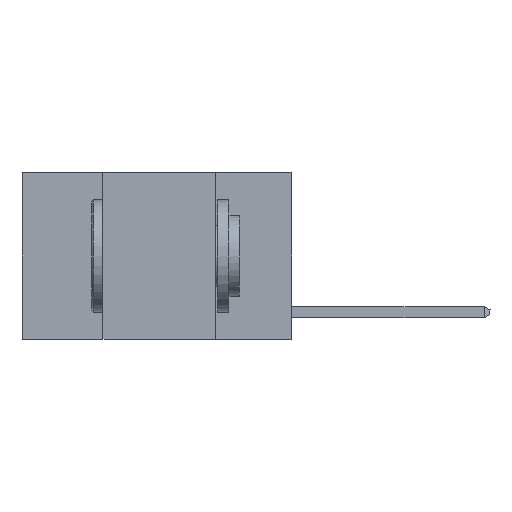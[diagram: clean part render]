
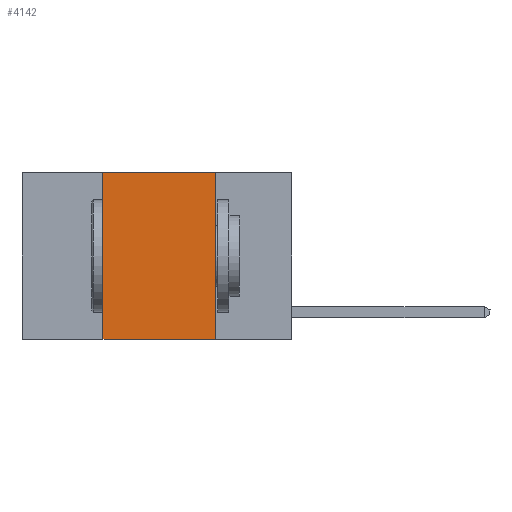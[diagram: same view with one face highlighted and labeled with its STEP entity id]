
A CAD part, left-side view. The second image highlights one B-rep face of the part: STEP entity #4142.
In plain terms, the highlighted planar face has unit normal (-1, 0, 0).
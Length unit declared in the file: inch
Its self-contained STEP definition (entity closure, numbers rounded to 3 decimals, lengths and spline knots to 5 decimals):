
#115 = CARTESIAN_POINT ( 'NONE',  ( 0., 0.6, 0. ) ) ;
#1295 = ORIENTED_EDGE ( 'NONE', *, *, #28066, .F. ) ;
#1952 = CARTESIAN_POINT ( 'NONE',  ( 0., 0.17, 0. ) ) ;
#2398 = DIRECTION ( 'NONE',  ( 0., -1., 0. ) ) ;
#3092 = CARTESIAN_POINT ( 'NONE',  ( 0., 0.6, -0.37 ) ) ;
#3655 = ORIENTED_EDGE ( 'NONE', *, *, #7582, .T. ) ;
#4142 = ADVANCED_FACE ( 'NONE', ( #26118 ), #16357, .F. ) ;
#4702 = EDGE_LOOP ( 'NONE', ( #1295, #19250, #13016, #3655 ) ) ;
#5059 = DIRECTION ( 'NONE',  ( 0., 0., -1. ) ) ;
#7136 = VERTEX_POINT ( 'NONE', #26392 ) ;
#7582 = EDGE_CURVE ( 'NONE', #7633, #23913, #25892, .T. ) ;
#7633 = VERTEX_POINT ( 'NONE', #21388 ) ;
#8542 = VECTOR ( 'NONE', #16693, 39.37008 ) ;
#8565 = CARTESIAN_POINT ( 'NONE',  ( 0., 0.42, 0. ) ) ;
#8942 = CARTESIAN_POINT ( 'NONE',  ( 0., 0.17, -0.37 ) ) ;
#9337 = EDGE_CURVE ( 'NONE', #7633, #23333, #25194, .T. ) ;
#11239 = CARTESIAN_POINT ( 'NONE',  ( 0., 0.42, 0. ) ) ;
#13016 = ORIENTED_EDGE ( 'NONE', *, *, #9337, .F. ) ;
#16357 = PLANE ( 'NONE',  #24434 ) ;
#16693 = DIRECTION ( 'NONE',  ( 0., -1., 0. ) ) ;
#18525 = CARTESIAN_POINT ( 'NONE',  ( 0., 0.6, 0. ) ) ;
#18625 = DIRECTION ( 'NONE',  ( 1., 0., 0. ) ) ;
#19250 = ORIENTED_EDGE ( 'NONE', *, *, #26886, .F. ) ;
#19489 = VECTOR ( 'NONE', #29016, 39.37008 ) ;
#20229 = LINE ( 'NONE', #1952, #19489 ) ;
#21388 = CARTESIAN_POINT ( 'NONE',  ( 0., 0.42, -0.37 ) ) ;
#23333 = VERTEX_POINT ( 'NONE', #11239 ) ;
#23491 = LINE ( 'NONE', #115, #28705 ) ;
#23913 = VERTEX_POINT ( 'NONE', #8942 ) ;
#24432 = DIRECTION ( 'NONE',  ( 0., 0., 1. ) ) ;
#24434 = AXIS2_PLACEMENT_3D ( 'NONE', #18525, #18625, #5059 ) ;
#25194 = LINE ( 'NONE', #8565, #26609 ) ;
#25892 = LINE ( 'NONE', #3092, #8542 ) ;
#26118 = FACE_OUTER_BOUND ( 'NONE', #4702, .T. ) ;
#26392 = CARTESIAN_POINT ( 'NONE',  ( 0., 0.17, 0. ) ) ;
#26609 = VECTOR ( 'NONE', #24432, 39.37008 ) ;
#26886 = EDGE_CURVE ( 'NONE', #23333, #7136, #23491, .T. ) ;
#28066 = EDGE_CURVE ( 'NONE', #7136, #23913, #20229, .T. ) ;
#28705 = VECTOR ( 'NONE', #2398, 39.37008 ) ;
#29016 = DIRECTION ( 'NONE',  ( 0., 0., -1. ) ) ;
